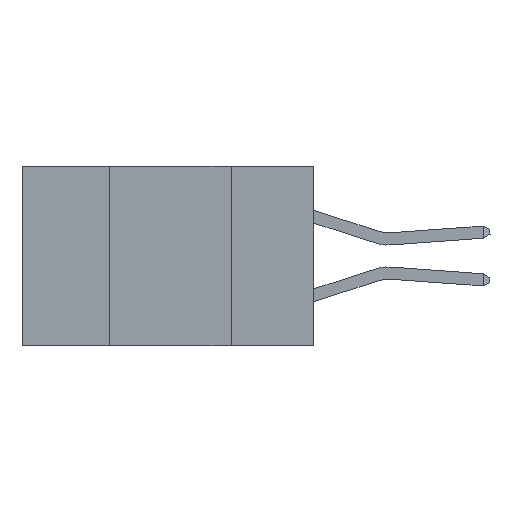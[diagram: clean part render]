
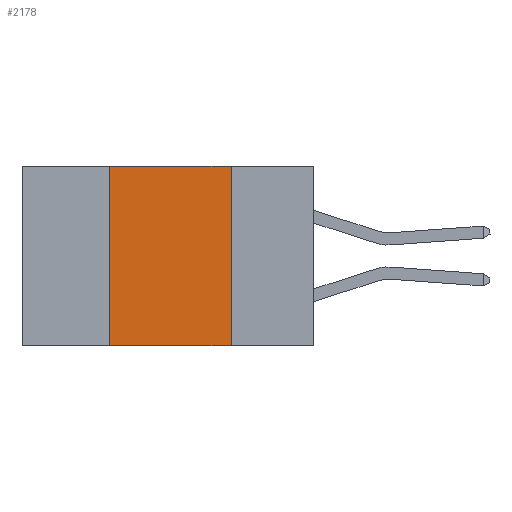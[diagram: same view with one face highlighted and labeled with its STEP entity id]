
A CAD part, left-side view. The second image highlights one B-rep face of the part: STEP entity #2178.
In plain terms, the highlighted planar face has unit normal (-1, 0, 0).
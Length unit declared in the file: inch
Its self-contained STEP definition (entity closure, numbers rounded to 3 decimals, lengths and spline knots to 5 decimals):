
#407 = DIRECTION ( 'NONE',  ( 0., 0., -1. ) ) ;
#425 = DIRECTION ( 'NONE',  ( 1., 0., 0. ) ) ;
#507 = EDGE_CURVE ( 'NONE', #5594, #8313, #3704, .T. ) ;
#664 = CARTESIAN_POINT ( 'NONE',  ( 0., 0.17, 0. ) ) ;
#694 = DIRECTION ( 'NONE',  ( 0., 0., 1. ) ) ;
#813 = VECTOR ( 'NONE', #694, 39.37008 ) ;
#1044 = ORIENTED_EDGE ( 'NONE', *, *, #10641, .F. ) ;
#1078 = ORIENTED_EDGE ( 'NONE', *, *, #7001, .F. ) ;
#1143 = ORIENTED_EDGE ( 'NONE', *, *, #507, .F. ) ;
#1169 = ORIENTED_EDGE ( 'NONE', *, *, #11447, .T. ) ;
#1833 = CARTESIAN_POINT ( 'NONE',  ( 0., 0.42, 0. ) ) ;
#1858 = PLANE ( 'NONE',  #13230 ) ;
#2178 = ADVANCED_FACE ( 'NONE', ( #11851 ), #1858, .F. ) ;
#2300 = VECTOR ( 'NONE', #10858, 39.37008 ) ;
#2616 = LINE ( 'NONE', #9820, #2300 ) ;
#2637 = LINE ( 'NONE', #11618, #10741 ) ;
#3704 = LINE ( 'NONE', #1833, #813 ) ;
#5289 = EDGE_LOOP ( 'NONE', ( #1044, #1078, #1143, #1169 ) ) ;
#5594 = VERTEX_POINT ( 'NONE', #8562 ) ;
#5612 = VERTEX_POINT ( 'NONE', #9222 ) ;
#5732 = CARTESIAN_POINT ( 'NONE',  ( 0., 0.6, 0. ) ) ;
#5750 = CARTESIAN_POINT ( 'NONE',  ( 0., 0.6, 0. ) ) ;
#7001 = EDGE_CURVE ( 'NONE', #8313, #7333, #12549, .T. ) ;
#7333 = VERTEX_POINT ( 'NONE', #664 ) ;
#8313 = VERTEX_POINT ( 'NONE', #11141 ) ;
#8562 = CARTESIAN_POINT ( 'NONE',  ( 0., 0.42, -0.37 ) ) ;
#9222 = CARTESIAN_POINT ( 'NONE',  ( 0., 0.17, -0.37 ) ) ;
#9774 = DIRECTION ( 'NONE',  ( 0., -1., 0. ) ) ;
#9820 = CARTESIAN_POINT ( 'NONE',  ( 0., 0.6, -0.37 ) ) ;
#10203 = VECTOR ( 'NONE', #9774, 39.37008 ) ;
#10641 = EDGE_CURVE ( 'NONE', #7333, #5612, #2637, .T. ) ;
#10741 = VECTOR ( 'NONE', #12617, 39.37008 ) ;
#10858 = DIRECTION ( 'NONE',  ( 0., -1., 0. ) ) ;
#11141 = CARTESIAN_POINT ( 'NONE',  ( 0., 0.42, 0. ) ) ;
#11447 = EDGE_CURVE ( 'NONE', #5594, #5612, #2616, .T. ) ;
#11618 = CARTESIAN_POINT ( 'NONE',  ( 0., 0.17, 0. ) ) ;
#11851 = FACE_OUTER_BOUND ( 'NONE', #5289, .T. ) ;
#12549 = LINE ( 'NONE', #5732, #10203 ) ;
#12617 = DIRECTION ( 'NONE',  ( 0., 0., -1. ) ) ;
#13230 = AXIS2_PLACEMENT_3D ( 'NONE', #5750, #425, #407 ) ;
